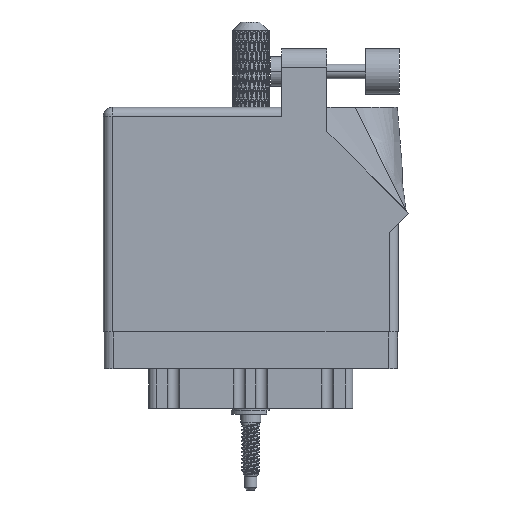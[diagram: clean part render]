
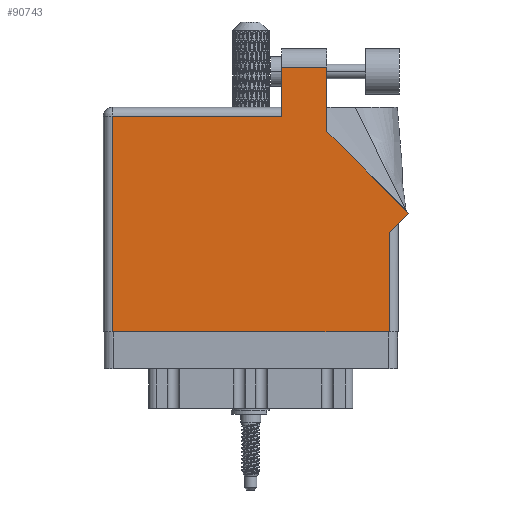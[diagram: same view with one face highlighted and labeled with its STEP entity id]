
A CAD part, front view. The second image highlights one B-rep face of the part: STEP entity #90743.
In plain terms, the highlighted face is planar.
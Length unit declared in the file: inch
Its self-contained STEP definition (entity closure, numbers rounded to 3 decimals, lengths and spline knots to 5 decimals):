
#5455 = CARTESIAN_POINT ( 'NONE',  ( 1.524, 1.36442, 0. ) ) ;
#6727 = LINE ( 'NONE', #71232, #97296 ) ;
#7818 = CARTESIAN_POINT ( 'NONE',  ( 0.062, 1.468, 0. ) ) ;
#7933 = EDGE_CURVE ( 'NONE', #77605, #63550, #69765, .T. ) ;
#8866 = DIRECTION ( 'NONE',  ( 0., -1., 0. ) ) ;
#10389 = VERTEX_POINT ( 'NONE', #28297 ) ;
#12268 = VECTOR ( 'NONE', #77121, 39.37008 ) ;
#13661 = LINE ( 'NONE', #29553, #12268 ) ;
#14902 = DIRECTION ( 'NONE',  ( 0., -1., 0. ) ) ;
#16343 = ORIENTED_EDGE ( 'NONE', *, *, #7933, .T. ) ;
#16470 = ORIENTED_EDGE ( 'NONE', *, *, #72384, .T. ) ;
#21157 = DIRECTION ( 'NONE',  ( -0.707, 0.707, 0. ) ) ;
#22004 = FACE_OUTER_BOUND ( 'NONE', #39748, .T. ) ;
#22452 = VERTEX_POINT ( 'NONE', #38860 ) ;
#23269 = ORIENTED_EDGE ( 'NONE', *, *, #89768, .T. ) ;
#23369 = VECTOR ( 'NONE', #21157, 39.37008 ) ;
#26042 = AXIS2_PLACEMENT_3D ( 'NONE', #73579, #29945, #29425 ) ;
#27432 = CARTESIAN_POINT ( 'NONE',  ( 2.08071, 0.80771, 0. ) ) ;
#28297 = CARTESIAN_POINT ( 'NONE',  ( 1.217, 1.468, 0. ) ) ;
#29425 = DIRECTION ( 'NONE',  ( -1., 0., 0. ) ) ;
#29553 = CARTESIAN_POINT ( 'NONE',  ( 0., 1.468, 0. ) ) ;
#29945 = DIRECTION ( 'NONE',  ( 0., 0., -1. ) ) ;
#30814 = VERTEX_POINT ( 'NONE', #53873 ) ;
#31365 = DIRECTION ( 'NONE',  ( 0., 1., 0. ) ) ;
#31531 = CARTESIAN_POINT ( 'NONE',  ( 2.01, 0.737, 0. ) ) ;
#31867 = CARTESIAN_POINT ( 'NONE',  ( 1.217, 1.805, 0. ) ) ;
#32103 = ORIENTED_EDGE ( 'NONE', *, *, #78479, .T. ) ;
#34695 = VECTOR ( 'NONE', #86489, 39.37008 ) ;
#35122 = EDGE_CURVE ( 'NONE', #68891, #10389, #74413, .T. ) ;
#36107 = LINE ( 'NONE', #68369, #57994 ) ;
#38585 = VECTOR ( 'NONE', #55755, 39.37008 ) ;
#38860 = CARTESIAN_POINT ( 'NONE',  ( 1.948, 0.675, 0. ) ) ;
#38989 = DIRECTION ( 'NONE',  ( 0., 1., 0. ) ) ;
#39748 = EDGE_LOOP ( 'NONE', ( #32103, #74591, #67522, #16470, #76693, #23269, #104305, #77078, #16343 ) ) ;
#44467 = VECTOR ( 'NONE', #14902, 39.37008 ) ;
#46811 = CARTESIAN_POINT ( 'NONE',  ( 1.524, 1.36442, 0. ) ) ;
#47119 = EDGE_CURVE ( 'NONE', #30814, #68891, #97460, .T. ) ;
#53873 = CARTESIAN_POINT ( 'NONE',  ( 1.524, 1.805, 0. ) ) ;
#55755 = DIRECTION ( 'NONE',  ( -1., 0., 0. ) ) ;
#57994 = VECTOR ( 'NONE', #92650, 39.37008 ) ;
#62648 = PLANE ( 'NONE',  #26042 ) ;
#63550 = VERTEX_POINT ( 'NONE', #46811 ) ;
#64387 = CARTESIAN_POINT ( 'NONE',  ( 1.217, 1.53, 0. ) ) ;
#65226 = CARTESIAN_POINT ( 'NONE',  ( 1.217, 1.805, 0. ) ) ;
#66645 = VECTOR ( 'NONE', #31365, 39.37008 ) ;
#66770 = VERTEX_POINT ( 'NONE', #72076 ) ;
#67522 = ORIENTED_EDGE ( 'NONE', *, *, #35122, .T. ) ;
#68369 = CARTESIAN_POINT ( 'NONE',  ( 0., 0., 0. ) ) ;
#68891 = VERTEX_POINT ( 'NONE', #31867 ) ;
#69765 = LINE ( 'NONE', #85627, #23369 ) ;
#70428 = LINE ( 'NONE', #78874, #44467 ) ;
#70449 = VECTOR ( 'NONE', #8866, 39.37008 ) ;
#71003 = LINE ( 'NONE', #5455, #66645 ) ;
#71232 = CARTESIAN_POINT ( 'NONE',  ( 1.948, 0.737, 0. ) ) ;
#72076 = CARTESIAN_POINT ( 'NONE',  ( 0.062, 0., 0. ) ) ;
#72384 = EDGE_CURVE ( 'NONE', #10389, #97811, #13661, .T. ) ;
#73579 = CARTESIAN_POINT ( 'NONE',  ( 0., 1.53, 0. ) ) ;
#74413 = LINE ( 'NONE', #64387, #70449 ) ;
#74591 = ORIENTED_EDGE ( 'NONE', *, *, #47119, .T. ) ;
#76693 = ORIENTED_EDGE ( 'NONE', *, *, #88402, .T. ) ;
#77078 = ORIENTED_EDGE ( 'NONE', *, *, #98843, .T. ) ;
#77121 = DIRECTION ( 'NONE',  ( -1., 0., 0. ) ) ;
#77605 = VERTEX_POINT ( 'NONE', #27432 ) ;
#78328 = CARTESIAN_POINT ( 'NONE',  ( 1.948, 0., 0. ) ) ;
#78479 = EDGE_CURVE ( 'NONE', #63550, #30814, #71003, .T. ) ;
#78586 = LINE ( 'NONE', #31531, #34695 ) ;
#78874 = CARTESIAN_POINT ( 'NONE',  ( 0.062, 0., 0. ) ) ;
#85627 = CARTESIAN_POINT ( 'NONE',  ( 2.08071, 0.80771, 0. ) ) ;
#86489 = DIRECTION ( 'NONE',  ( 0.707, 0.707, 0. ) ) ;
#87105 = VERTEX_POINT ( 'NONE', #78328 ) ;
#88402 = EDGE_CURVE ( 'NONE', #97811, #66770, #70428, .T. ) ;
#89768 = EDGE_CURVE ( 'NONE', #66770, #87105, #36107, .T. ) ;
#90743 = ADVANCED_FACE ( 'NONE', ( #22004 ), #62648, .F. ) ;
#92650 = DIRECTION ( 'NONE',  ( 1., 0., 0. ) ) ;
#97296 = VECTOR ( 'NONE', #38989, 39.37008 ) ;
#97460 = LINE ( 'NONE', #65226, #38585 ) ;
#97811 = VERTEX_POINT ( 'NONE', #7818 ) ;
#98843 = EDGE_CURVE ( 'NONE', #22452, #77605, #78586, .T. ) ;
#101187 = EDGE_CURVE ( 'NONE', #87105, #22452, #6727, .T. ) ;
#104305 = ORIENTED_EDGE ( 'NONE', *, *, #101187, .T. ) ;
